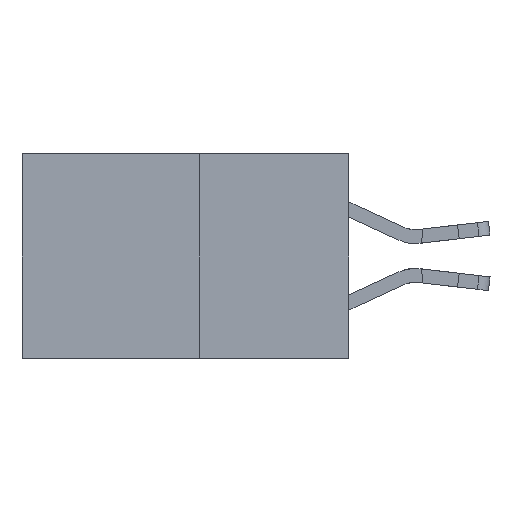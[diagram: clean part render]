
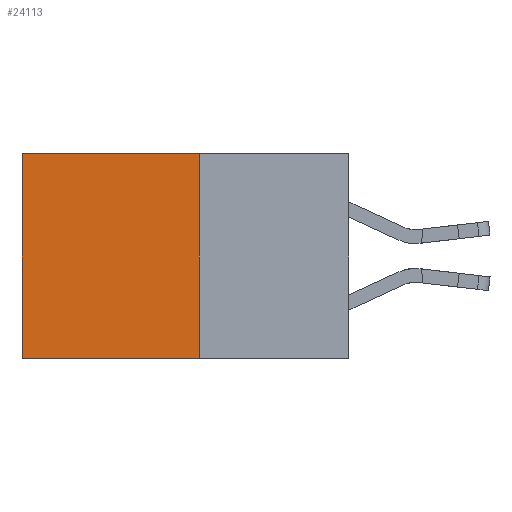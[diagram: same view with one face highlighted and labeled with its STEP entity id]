
A CAD part, left-side view. The second image highlights one B-rep face of the part: STEP entity #24113.
In plain terms, the highlighted planar face has unit normal (-1, 0, 0).
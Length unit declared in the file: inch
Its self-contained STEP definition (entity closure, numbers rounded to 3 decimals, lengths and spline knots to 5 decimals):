
#250 = DIRECTION ( 'NONE',  ( 0., 1., 0. ) ) ;
#382 = EDGE_CURVE ( 'NONE', #20208, #4330, #9736, .T. ) ;
#533 = EDGE_CURVE ( 'NONE', #19435, #4330, #7217, .T. ) ;
#1318 = VERTEX_POINT ( 'NONE', #2126 ) ;
#2053 = CARTESIAN_POINT ( 'NONE',  ( 0.277, 0.59, -0.37 ) ) ;
#2126 = CARTESIAN_POINT ( 'NONE',  ( 0.277, 0.27, 0. ) ) ;
#3903 = CARTESIAN_POINT ( 'NONE',  ( 0.277, 0.27, -0.37 ) ) ;
#4056 = CARTESIAN_POINT ( 'NONE',  ( 0.277, 0.27, 0. ) ) ;
#4330 = VERTEX_POINT ( 'NONE', #21892 ) ;
#5588 = CARTESIAN_POINT ( 'NONE',  ( 0.277, 0.27, -0.37 ) ) ;
#5719 = ORIENTED_EDGE ( 'NONE', *, *, #533, .F. ) ;
#5862 = PLANE ( 'NONE',  #24967 ) ;
#6582 = VECTOR ( 'NONE', #11254, 39.37008 ) ;
#6786 = EDGE_CURVE ( 'NONE', #1318, #20208, #18603, .T. ) ;
#7217 = LINE ( 'NONE', #22730, #6582 ) ;
#7700 = VECTOR ( 'NONE', #250, 39.37008 ) ;
#7800 = ORIENTED_EDGE ( 'NONE', *, *, #13254, .F. ) ;
#8079 = ORIENTED_EDGE ( 'NONE', *, *, #382, .T. ) ;
#9736 = LINE ( 'NONE', #2053, #20607 ) ;
#9935 = DIRECTION ( 'NONE',  ( 1., 0., 0. ) ) ;
#10441 = FACE_OUTER_BOUND ( 'NONE', #14419, .T. ) ;
#11254 = DIRECTION ( 'NONE',  ( 0., 1., 0. ) ) ;
#13254 = EDGE_CURVE ( 'NONE', #1318, #19435, #16958, .T. ) ;
#14419 = EDGE_LOOP ( 'NONE', ( #8079, #5719, #7800, #15301 ) ) ;
#15301 = ORIENTED_EDGE ( 'NONE', *, *, #6786, .T. ) ;
#16058 = CARTESIAN_POINT ( 'NONE',  ( 0.277, 0.59, 0. ) ) ;
#16958 = LINE ( 'NONE', #3903, #21643 ) ;
#18603 = LINE ( 'NONE', #4056, #7700 ) ;
#19435 = VERTEX_POINT ( 'NONE', #5588 ) ;
#19776 = DIRECTION ( 'NONE',  ( 0., 0., -1. ) ) ;
#20142 = CARTESIAN_POINT ( 'NONE',  ( 0.277, 0.27, -0.37 ) ) ;
#20208 = VERTEX_POINT ( 'NONE', #16058 ) ;
#20242 = DIRECTION ( 'NONE',  ( 0., 0., -1. ) ) ;
#20607 = VECTOR ( 'NONE', #19776, 39.37008 ) ;
#21643 = VECTOR ( 'NONE', #20242, 39.37008 ) ;
#21892 = CARTESIAN_POINT ( 'NONE',  ( 0.277, 0.59, -0.37 ) ) ;
#22730 = CARTESIAN_POINT ( 'NONE',  ( 0.277, 0.27, -0.37 ) ) ;
#24075 = DIRECTION ( 'NONE',  ( 0., 0., -1. ) ) ;
#24113 = ADVANCED_FACE ( 'NONE', ( #10441 ), #5862, .F. ) ;
#24967 = AXIS2_PLACEMENT_3D ( 'NONE', #20142, #9935, #24075 ) ;
